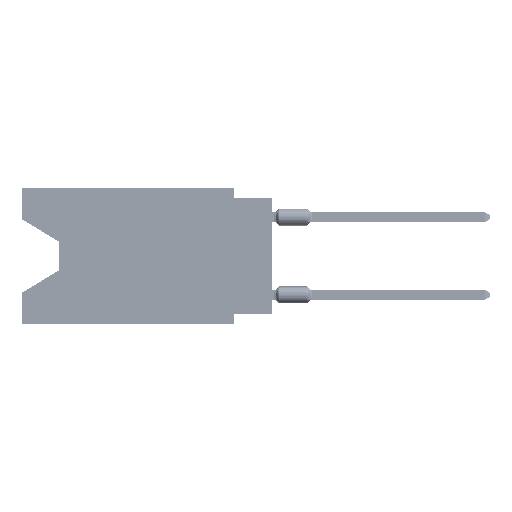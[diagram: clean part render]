
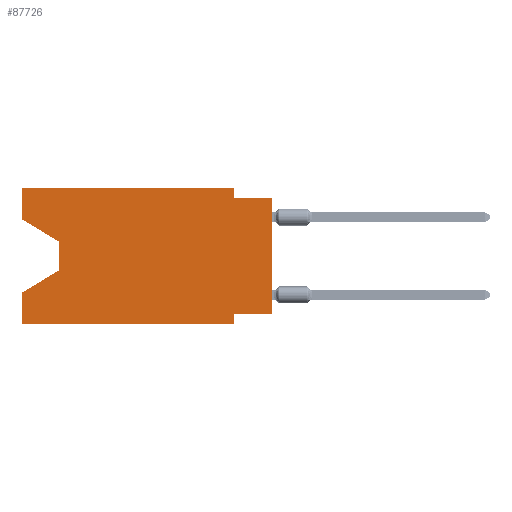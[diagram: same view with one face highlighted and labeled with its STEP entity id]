
A CAD part, left-side view. The second image highlights one B-rep face of the part: STEP entity #87726.
In plain terms, the highlighted planar face has unit normal (-1, 0, 0).
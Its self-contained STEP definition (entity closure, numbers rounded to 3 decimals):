
#3493 = VERTEX_POINT ( 'NONE', #78434 ) ;
#5918 = LINE ( 'NONE', #36696, #78087 ) ;
#7560 = ORIENTED_EDGE ( 'NONE', *, *, #55547, .F. ) ;
#8015 = FACE_OUTER_BOUND ( 'NONE', #22125, .T. ) ;
#8701 = LINE ( 'NONE', #25403, #11012 ) ;
#10814 = ORIENTED_EDGE ( 'NONE', *, *, #16469, .F. ) ;
#11012 = VECTOR ( 'NONE', #88062, 1000. ) ;
#11440 = DIRECTION ( 'NONE',  ( 0., 0.855, -0.519 ) ) ;
#11563 = EDGE_CURVE ( 'NONE', #33101, #64325, #28578, .T. ) ;
#11771 = CARTESIAN_POINT ( 'NONE',  ( 0., 2.54, 0. ) ) ;
#12415 = DIRECTION ( 'NONE',  ( 0., 0., 1. ) ) ;
#13187 = CARTESIAN_POINT ( 'NONE',  ( 0., 0., -0.635 ) ) ;
#16099 = CARTESIAN_POINT ( 'NONE',  ( 0., 16.383, -8.89 ) ) ;
#16469 = EDGE_CURVE ( 'NONE', #26657, #76668, #40630, .T. ) ;
#17540 = DIRECTION ( 'NONE',  ( 0., 0., -1. ) ) ;
#20199 = VERTEX_POINT ( 'NONE', #13187 ) ;
#21206 = EDGE_CURVE ( 'NONE', #91142, #24503, #76446, .T. ) ;
#22125 = EDGE_LOOP ( 'NONE', ( #32207, #87234, #25440, #47818, #96035, #10814, #7560, #68047, #73056, #51599, #28807, #66290 ) ) ;
#22653 = CARTESIAN_POINT ( 'NONE',  ( 0., 16.383, -2.038 ) ) ;
#24503 = VERTEX_POINT ( 'NONE', #69075 ) ;
#25403 = CARTESIAN_POINT ( 'NONE',  ( 0., 0., 0. ) ) ;
#25440 = ORIENTED_EDGE ( 'NONE', *, *, #69951, .T. ) ;
#25566 = CARTESIAN_POINT ( 'NONE',  ( 0., 13.97, -5.385 ) ) ;
#26657 = VERTEX_POINT ( 'NONE', #71064 ) ;
#27059 = LINE ( 'NONE', #28102, #44545 ) ;
#27203 = CARTESIAN_POINT ( 'NONE',  ( 0., 0., -0.635 ) ) ;
#28102 = CARTESIAN_POINT ( 'NONE',  ( 0., 16.383, 0. ) ) ;
#28578 = LINE ( 'NONE', #83936, #100070 ) ;
#28807 = ORIENTED_EDGE ( 'NONE', *, *, #83455, .F. ) ;
#28921 = VERTEX_POINT ( 'NONE', #11771 ) ;
#32207 = ORIENTED_EDGE ( 'NONE', *, *, #21206, .T. ) ;
#33101 = VERTEX_POINT ( 'NONE', #63260 ) ;
#36696 = CARTESIAN_POINT ( 'NONE',  ( 0., 2.54, 0. ) ) ;
#36745 = DIRECTION ( 'NONE',  ( 0., -0.855, -0.519 ) ) ;
#37748 = AXIS2_PLACEMENT_3D ( 'NONE', #86372, #48177, #79049 ) ;
#38105 = LINE ( 'NONE', #76255, #43929 ) ;
#38518 = VERTEX_POINT ( 'NONE', #55746 ) ;
#40630 = LINE ( 'NONE', #73023, #58131 ) ;
#41715 = LINE ( 'NONE', #25566, #54303 ) ;
#42428 = VECTOR ( 'NONE', #17540, 1000. ) ;
#43446 = CARTESIAN_POINT ( 'NONE',  ( 0., 0., -8.255 ) ) ;
#43929 = VECTOR ( 'NONE', #61614, 1000. ) ;
#44530 = DIRECTION ( 'NONE',  ( 0., 0., -1. ) ) ;
#44545 = VECTOR ( 'NONE', #84475, 1000. ) ;
#47818 = ORIENTED_EDGE ( 'NONE', *, *, #11563, .F. ) ;
#48177 = DIRECTION ( 'NONE',  ( 1., 0., 0. ) ) ;
#50247 = DIRECTION ( 'NONE',  ( 0., 1., 0. ) ) ;
#50374 = VECTOR ( 'NONE', #50247, 1000. ) ;
#51599 = ORIENTED_EDGE ( 'NONE', *, *, #74591, .F. ) ;
#51852 = CARTESIAN_POINT ( 'NONE',  ( 0., 2.54, -0.635 ) ) ;
#53278 = LINE ( 'NONE', #27203, #92324 ) ;
#54303 = VECTOR ( 'NONE', #11440, 1000. ) ;
#55248 = DIRECTION ( 'NONE',  ( 0., -1., 0. ) ) ;
#55547 = EDGE_CURVE ( 'NONE', #38518, #26657, #91499, .T. ) ;
#55746 = CARTESIAN_POINT ( 'NONE',  ( 0., 0., -8.255 ) ) ;
#58131 = VECTOR ( 'NONE', #64137, 1000. ) ;
#58566 = CARTESIAN_POINT ( 'NONE',  ( 0., 16.383, 0. ) ) ;
#59611 = CARTESIAN_POINT ( 'NONE',  ( 0., 2.54, -8.89 ) ) ;
#61614 = DIRECTION ( 'NONE',  ( 0., -1., 0. ) ) ;
#63260 = CARTESIAN_POINT ( 'NONE',  ( 0., 16.383, -8.89 ) ) ;
#64137 = DIRECTION ( 'NONE',  ( 0., 0., -1. ) ) ;
#64325 = VERTEX_POINT ( 'NONE', #95957 ) ;
#66290 = ORIENTED_EDGE ( 'NONE', *, *, #100151, .F. ) ;
#68047 = ORIENTED_EDGE ( 'NONE', *, *, #100374, .T. ) ;
#68580 = VECTOR ( 'NONE', #36745, 1000. ) ;
#69075 = CARTESIAN_POINT ( 'NONE',  ( 0., 13.97, -3.505 ) ) ;
#69951 = EDGE_CURVE ( 'NONE', #3493, #64325, #41715, .T. ) ;
#70213 = VECTOR ( 'NONE', #55248, 1000. ) ;
#71064 = CARTESIAN_POINT ( 'NONE',  ( 0., 2.54, -8.255 ) ) ;
#72411 = VERTEX_POINT ( 'NONE', #58566 ) ;
#73023 = CARTESIAN_POINT ( 'NONE',  ( 0., 2.54, -8.89 ) ) ;
#73056 = ORIENTED_EDGE ( 'NONE', *, *, #85098, .F. ) ;
#74591 = EDGE_CURVE ( 'NONE', #28921, #83073, #5918, .T. ) ;
#75474 = CARTESIAN_POINT ( 'NONE',  ( 0., 16.383, -2.038 ) ) ;
#76255 = CARTESIAN_POINT ( 'NONE',  ( 0., 16.383, 0. ) ) ;
#76446 = LINE ( 'NONE', #22653, #68580 ) ;
#76668 = VERTEX_POINT ( 'NONE', #59611 ) ;
#78087 = VECTOR ( 'NONE', #44530, 1000. ) ;
#78434 = CARTESIAN_POINT ( 'NONE',  ( 0., 13.97, -5.385 ) ) ;
#79049 = DIRECTION ( 'NONE',  ( 0., 0., -1. ) ) ;
#80870 = EDGE_CURVE ( 'NONE', #33101, #76668, #94950, .T. ) ;
#83073 = VERTEX_POINT ( 'NONE', #51852 ) ;
#83455 = EDGE_CURVE ( 'NONE', #72411, #28921, #38105, .T. ) ;
#83936 = CARTESIAN_POINT ( 'NONE',  ( 0., 16.383, 0. ) ) ;
#84475 = DIRECTION ( 'NONE',  ( 0., 0., 1. ) ) ;
#85098 = EDGE_CURVE ( 'NONE', #83073, #20199, #53278, .T. ) ;
#86323 = EDGE_CURVE ( 'NONE', #24503, #3493, #89066, .T. ) ;
#86372 = CARTESIAN_POINT ( 'NONE',  ( 0., 16.383, 0. ) ) ;
#87234 = ORIENTED_EDGE ( 'NONE', *, *, #86323, .T. ) ;
#87726 = ADVANCED_FACE ( 'NONE', ( #8015 ), #94710, .F. ) ;
#88062 = DIRECTION ( 'NONE',  ( 0., 0., 1. ) ) ;
#88539 = CARTESIAN_POINT ( 'NONE',  ( 0., 13.97, -3.505 ) ) ;
#89066 = LINE ( 'NONE', #88539, #42428 ) ;
#90898 = DIRECTION ( 'NONE',  ( 0., -1., 0. ) ) ;
#91142 = VERTEX_POINT ( 'NONE', #75474 ) ;
#91499 = LINE ( 'NONE', #43446, #50374 ) ;
#92324 = VECTOR ( 'NONE', #90898, 1000. ) ;
#94710 = PLANE ( 'NONE',  #37748 ) ;
#94950 = LINE ( 'NONE', #16099, #70213 ) ;
#95957 = CARTESIAN_POINT ( 'NONE',  ( 0., 16.383, -6.852 ) ) ;
#96035 = ORIENTED_EDGE ( 'NONE', *, *, #80870, .T. ) ;
#100070 = VECTOR ( 'NONE', #12415, 1000. ) ;
#100151 = EDGE_CURVE ( 'NONE', #91142, #72411, #27059, .T. ) ;
#100374 = EDGE_CURVE ( 'NONE', #38518, #20199, #8701, .T. ) ;
